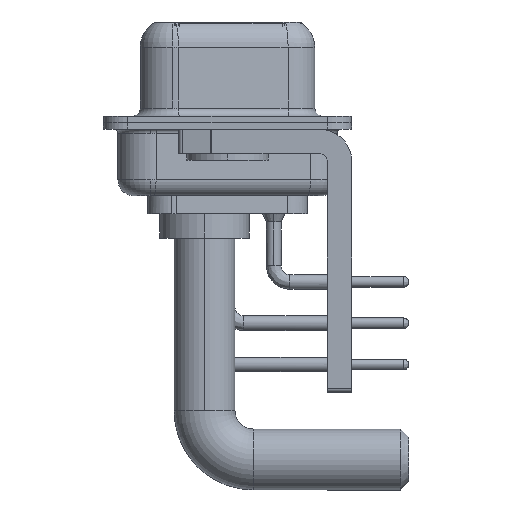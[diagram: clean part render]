
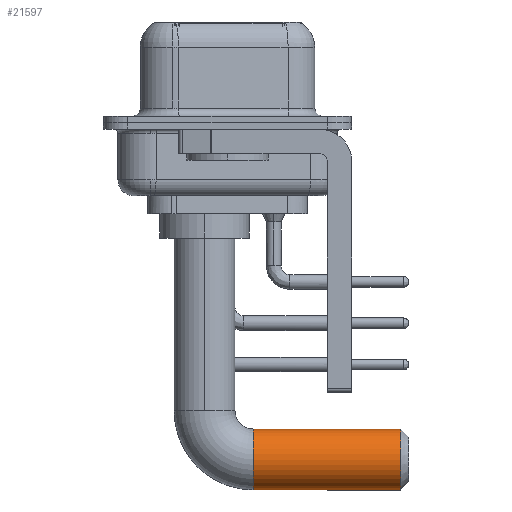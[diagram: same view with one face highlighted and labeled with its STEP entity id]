
A CAD part, left-side view. The second image highlights one B-rep face of the part: STEP entity #21597.
In plain terms, the highlighted cylindrical face has radius 1.875 mm (diameter 3.75 mm), a partial arc.
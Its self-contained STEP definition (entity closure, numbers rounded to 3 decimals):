
#521 = FACE_OUTER_BOUND ( 'NONE', #26959, .T. ) ;
#693 = VERTEX_POINT ( 'NONE', #20414 ) ;
#1017 = CARTESIAN_POINT ( 'NONE',  ( 0., -3., -13.63 ) ) ;
#1456 = CARTESIAN_POINT ( 'NONE',  ( 0., -3., -15.505 ) ) ;
#1479 = DIRECTION ( 'NONE',  ( 0., 0., -1. ) ) ;
#2070 = EDGE_CURVE ( 'NONE', #25972, #693, #32320, .T. ) ;
#3527 = CARTESIAN_POINT ( 'NONE',  ( 0., -12.07, -11.755 ) ) ;
#4175 = CARTESIAN_POINT ( 'NONE',  ( 0., -12.07, -13.63 ) ) ;
#4197 = ORIENTED_EDGE ( 'NONE', *, *, #2070, .T. ) ;
#5007 = ORIENTED_EDGE ( 'NONE', *, *, #32071, .F. ) ;
#6089 = DIRECTION ( 'NONE',  ( 0., 0., -1. ) ) ;
#6858 = LINE ( 'NONE', #1456, #25091 ) ;
#7940 = AXIS2_PLACEMENT_3D ( 'NONE', #1017, #16505, #6089 ) ;
#8085 = ORIENTED_EDGE ( 'NONE', *, *, #9054, .T. ) ;
#8486 = VERTEX_POINT ( 'NONE', #3527 ) ;
#9054 = EDGE_CURVE ( 'NONE', #693, #12623, #6858, .T. ) ;
#10700 = CARTESIAN_POINT ( 'NONE',  ( 0., -12.07, -15.505 ) ) ;
#10824 = CYLINDRICAL_SURFACE ( 'NONE', #7940, 1.875 ) ;
#11426 = ORIENTED_EDGE ( 'NONE', *, *, #33260, .T. ) ;
#12623 = VERTEX_POINT ( 'NONE', #10700 ) ;
#14013 = VECTOR ( 'NONE', #16171, 1000. ) ;
#15046 = CARTESIAN_POINT ( 'NONE',  ( 0., -3., -13.63 ) ) ;
#16171 = DIRECTION ( 'NONE',  ( 0., -1., 0. ) ) ;
#16489 = CARTESIAN_POINT ( 'NONE',  ( 0., -3., -11.755 ) ) ;
#16505 = DIRECTION ( 'NONE',  ( 0., -1., 0. ) ) ;
#17466 = DIRECTION ( 'NONE',  ( 0., -1., 0. ) ) ;
#20255 = DIRECTION ( 'NONE',  ( 0., -1., 0. ) ) ;
#20414 = CARTESIAN_POINT ( 'NONE',  ( 0., -3., -15.505 ) ) ;
#21597 = ADVANCED_FACE ( 'NONE', ( #521 ), #10824, .T. ) ;
#25091 = VECTOR ( 'NONE', #17466, 1000. ) ;
#25361 = CIRCLE ( 'NONE', #26976, 1.875 ) ;
#25972 = VERTEX_POINT ( 'NONE', #30603 ) ;
#26408 = AXIS2_PLACEMENT_3D ( 'NONE', #15046, #20255, #33233 ) ;
#26959 = EDGE_LOOP ( 'NONE', ( #5007, #4197, #8085, #11426 ) ) ;
#26976 = AXIS2_PLACEMENT_3D ( 'NONE', #4175, #32626, #1479 ) ;
#29434 = LINE ( 'NONE', #16489, #14013 ) ;
#30603 = CARTESIAN_POINT ( 'NONE',  ( 0., -3., -11.755 ) ) ;
#32071 = EDGE_CURVE ( 'NONE', #25972, #8486, #29434, .T. ) ;
#32320 = CIRCLE ( 'NONE', #26408, 1.875 ) ;
#32626 = DIRECTION ( 'NONE',  ( 0., 1., 0. ) ) ;
#33233 = DIRECTION ( 'NONE',  ( -1., 0., 0. ) ) ;
#33260 = EDGE_CURVE ( 'NONE', #12623, #8486, #25361, .T. ) ;
